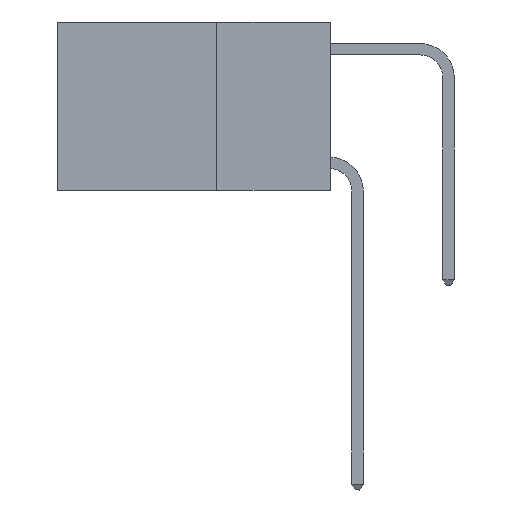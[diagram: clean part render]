
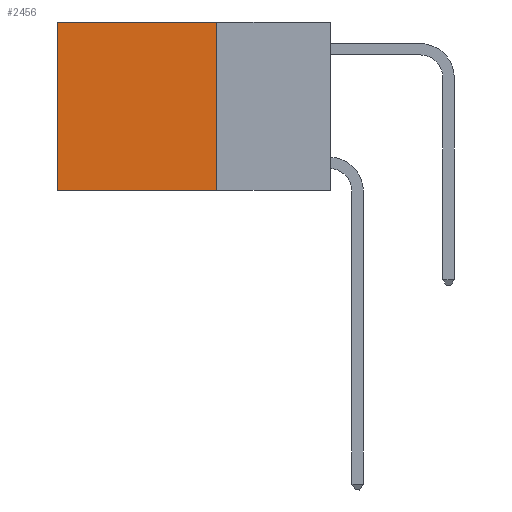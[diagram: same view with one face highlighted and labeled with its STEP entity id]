
A CAD part, left-side view. The second image highlights one B-rep face of the part: STEP entity #2456.
In plain terms, the highlighted planar face has unit normal (-1, 0, 0).
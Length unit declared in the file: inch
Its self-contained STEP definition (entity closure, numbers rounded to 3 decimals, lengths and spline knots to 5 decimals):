
#692 = CARTESIAN_POINT ( 'NONE',  ( 0.2625, 0.25, 0. ) ) ;
#847 = LINE ( 'NONE', #22556, #5907 ) ;
#1836 = CARTESIAN_POINT ( 'NONE',  ( 0.2625, 0.6, 0. ) ) ;
#2456 = ADVANCED_FACE ( 'NONE', ( #15331 ), #21606, .F. ) ;
#3155 = CARTESIAN_POINT ( 'NONE',  ( 0.2625, 0.6, 0. ) ) ;
#3750 = VECTOR ( 'NONE', #14086, 39.37008 ) ;
#5032 = DIRECTION ( 'NONE',  ( 0., 0., -1. ) ) ;
#5791 = VERTEX_POINT ( 'NONE', #17135 ) ;
#5907 = VECTOR ( 'NONE', #11234, 39.37008 ) ;
#6981 = VECTOR ( 'NONE', #14399, 39.37008 ) ;
#8005 = ORIENTED_EDGE ( 'NONE', *, *, #9077, .F. ) ;
#9077 = EDGE_CURVE ( 'NONE', #14756, #5791, #18299, .T. ) ;
#10049 = EDGE_CURVE ( 'NONE', #5791, #23587, #17079, .T. ) ;
#10142 = ORIENTED_EDGE ( 'NONE', *, *, #19588, .T. ) ;
#10253 = CARTESIAN_POINT ( 'NONE',  ( 0.2625, 0.25, 0. ) ) ;
#11234 = DIRECTION ( 'NONE',  ( 0., 1., 0. ) ) ;
#12184 = DIRECTION ( 'NONE',  ( 0., 0., -1. ) ) ;
#12552 = CARTESIAN_POINT ( 'NONE',  ( 0.2625, 0.6, -0.37 ) ) ;
#14086 = DIRECTION ( 'NONE',  ( 0., 0., -1. ) ) ;
#14399 = DIRECTION ( 'NONE',  ( 0., 1., 0. ) ) ;
#14756 = VERTEX_POINT ( 'NONE', #18150 ) ;
#15331 = FACE_OUTER_BOUND ( 'NONE', #21927, .T. ) ;
#16369 = VECTOR ( 'NONE', #5032, 39.37008 ) ;
#16380 = CARTESIAN_POINT ( 'NONE',  ( 0.2625, 0.25, -0.37 ) ) ;
#16601 = ORIENTED_EDGE ( 'NONE', *, *, #18647, .T. ) ;
#17079 = LINE ( 'NONE', #16380, #6981 ) ;
#17135 = CARTESIAN_POINT ( 'NONE',  ( 0.2625, 0.25, -0.37 ) ) ;
#18150 = CARTESIAN_POINT ( 'NONE',  ( 0.2625, 0.25, 0. ) ) ;
#18299 = LINE ( 'NONE', #692, #3750 ) ;
#18647 = EDGE_CURVE ( 'NONE', #21532, #23587, #20164, .T. ) ;
#19588 = EDGE_CURVE ( 'NONE', #14756, #21532, #847, .T. ) ;
#20164 = LINE ( 'NONE', #3155, #16369 ) ;
#20608 = AXIS2_PLACEMENT_3D ( 'NONE', #10253, #23499, #12184 ) ;
#21532 = VERTEX_POINT ( 'NONE', #1836 ) ;
#21606 = PLANE ( 'NONE',  #20608 ) ;
#21927 = EDGE_LOOP ( 'NONE', ( #16601, #23027, #8005, #10142 ) ) ;
#22556 = CARTESIAN_POINT ( 'NONE',  ( 0.2625, 0.25, 0. ) ) ;
#23027 = ORIENTED_EDGE ( 'NONE', *, *, #10049, .F. ) ;
#23499 = DIRECTION ( 'NONE',  ( 1., 0., 0. ) ) ;
#23587 = VERTEX_POINT ( 'NONE', #12552 ) ;
